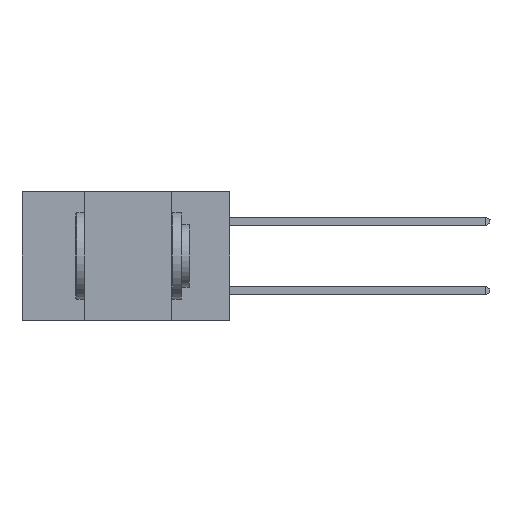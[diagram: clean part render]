
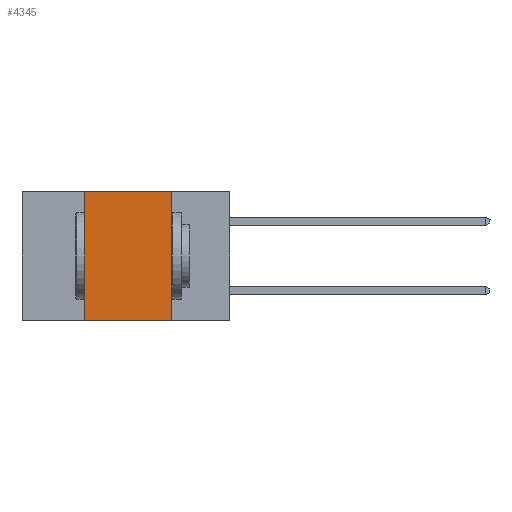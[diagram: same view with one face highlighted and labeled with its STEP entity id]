
A CAD part, left-side view. The second image highlights one B-rep face of the part: STEP entity #4345.
In plain terms, the highlighted planar face has unit normal (-1, 0, 0).
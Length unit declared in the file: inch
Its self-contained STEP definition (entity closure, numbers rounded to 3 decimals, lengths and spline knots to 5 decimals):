
#118 = CARTESIAN_POINT ( 'NONE',  ( 0., 0.17, -0.37 ) ) ;
#485 = LINE ( 'NONE', #17275, #13667 ) ;
#513 = DIRECTION ( 'NONE',  ( 1., 0., 0. ) ) ;
#845 = EDGE_CURVE ( 'NONE', #5306, #2085, #8399, .T. ) ;
#1199 = ORIENTED_EDGE ( 'NONE', *, *, #845, .F. ) ;
#1237 = LINE ( 'NONE', #6760, #15041 ) ;
#1267 = ORIENTED_EDGE ( 'NONE', *, *, #11109, .T. ) ;
#1661 = LINE ( 'NONE', #5750, #12623 ) ;
#1919 = CARTESIAN_POINT ( 'NONE',  ( 0., 0.42, 0. ) ) ;
#2085 = VERTEX_POINT ( 'NONE', #118 ) ;
#2910 = EDGE_CURVE ( 'NONE', #9329, #17046, #1237, .T. ) ;
#3113 = ORIENTED_EDGE ( 'NONE', *, *, #6720, .F. ) ;
#4345 = ADVANCED_FACE ( 'NONE', ( #12699 ), #11014, .F. ) ;
#5306 = VERTEX_POINT ( 'NONE', #12664 ) ;
#5608 = DIRECTION ( 'NONE',  ( 0., 0., -1. ) ) ;
#5750 = CARTESIAN_POINT ( 'NONE',  ( 0., 0.6, -0.37 ) ) ;
#5767 = CARTESIAN_POINT ( 'NONE',  ( 0., 0.42, -0.37 ) ) ;
#6720 = EDGE_CURVE ( 'NONE', #17046, #5306, #485, .T. ) ;
#6760 = CARTESIAN_POINT ( 'NONE',  ( 0., 0.42, -0.37 ) ) ;
#8399 = LINE ( 'NONE', #12470, #10537 ) ;
#8710 = CARTESIAN_POINT ( 'NONE',  ( 0., 0.6, 0. ) ) ;
#9099 = AXIS2_PLACEMENT_3D ( 'NONE', #8710, #513, #5608 ) ;
#9191 = DIRECTION ( 'NONE',  ( 0., -1., 0. ) ) ;
#9250 = DIRECTION ( 'NONE',  ( 0., 0., 1. ) ) ;
#9329 = VERTEX_POINT ( 'NONE', #5767 ) ;
#10537 = VECTOR ( 'NONE', #12556, 39.37008 ) ;
#10866 = EDGE_LOOP ( 'NONE', ( #1199, #3113, #13864, #1267 ) ) ;
#10992 = DIRECTION ( 'NONE',  ( 0., -1., 0. ) ) ;
#11014 = PLANE ( 'NONE',  #9099 ) ;
#11109 = EDGE_CURVE ( 'NONE', #9329, #2085, #1661, .T. ) ;
#12470 = CARTESIAN_POINT ( 'NONE',  ( 0., 0.17, -0.37 ) ) ;
#12556 = DIRECTION ( 'NONE',  ( 0., 0., -1. ) ) ;
#12623 = VECTOR ( 'NONE', #10992, 39.37008 ) ;
#12664 = CARTESIAN_POINT ( 'NONE',  ( 0., 0.17, 0. ) ) ;
#12699 = FACE_OUTER_BOUND ( 'NONE', #10866, .T. ) ;
#13667 = VECTOR ( 'NONE', #9191, 39.37008 ) ;
#13864 = ORIENTED_EDGE ( 'NONE', *, *, #2910, .F. ) ;
#15041 = VECTOR ( 'NONE', #9250, 39.37008 ) ;
#17046 = VERTEX_POINT ( 'NONE', #1919 ) ;
#17275 = CARTESIAN_POINT ( 'NONE',  ( 0., 0.6, 0. ) ) ;
